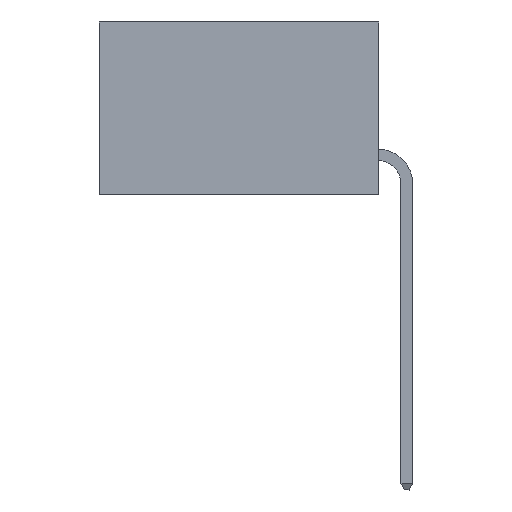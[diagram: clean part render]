
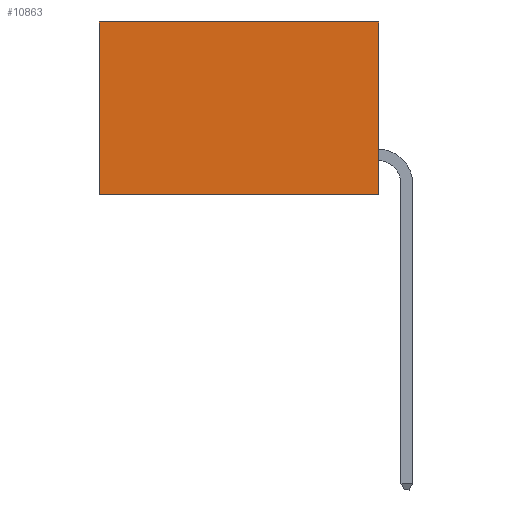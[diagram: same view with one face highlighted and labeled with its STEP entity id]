
A CAD part, left-side view. The second image highlights one B-rep face of the part: STEP entity #10863.
In plain terms, the highlighted planar face has unit normal (-1, 0, 0).
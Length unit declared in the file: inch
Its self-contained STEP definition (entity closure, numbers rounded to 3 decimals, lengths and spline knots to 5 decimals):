
#72 = CARTESIAN_POINT ( 'NONE',  ( 0.298, 0., -0.37 ) ) ;
#429 = DIRECTION ( 'NONE',  ( 0., 0., -1. ) ) ;
#1013 = VERTEX_POINT ( 'NONE', #72 ) ;
#1356 = VERTEX_POINT ( 'NONE', #2576 ) ;
#2576 = CARTESIAN_POINT ( 'NONE',  ( 0.298, 0.6, -0.37 ) ) ;
#2597 = DIRECTION ( 'NONE',  ( 0., 1., 0. ) ) ;
#3176 = VERTEX_POINT ( 'NONE', #16357 ) ;
#3367 = EDGE_CURVE ( 'NONE', #12695, #3176, #22529, .T. ) ;
#4934 = PLANE ( 'NONE',  #14690 ) ;
#4949 = EDGE_LOOP ( 'NONE', ( #16089, #23183, #5332, #28671 ) ) ;
#5332 = ORIENTED_EDGE ( 'NONE', *, *, #9638, .F. ) ;
#6008 = CARTESIAN_POINT ( 'NONE',  ( 0.298, 0., -0.37 ) ) ;
#7789 = DIRECTION ( 'NONE',  ( 0., 0., -1. ) ) ;
#9040 = VECTOR ( 'NONE', #7789, 39.37008 ) ;
#9498 = DIRECTION ( 'NONE',  ( 1., 0., 0. ) ) ;
#9638 = EDGE_CURVE ( 'NONE', #12695, #1013, #15044, .T. ) ;
#10863 = ADVANCED_FACE ( 'NONE', ( #22324 ), #4934, .F. ) ;
#12443 = VECTOR ( 'NONE', #15086, 39.37008 ) ;
#12695 = VERTEX_POINT ( 'NONE', #15808 ) ;
#14014 = EDGE_CURVE ( 'NONE', #1013, #1356, #24351, .T. ) ;
#14690 = AXIS2_PLACEMENT_3D ( 'NONE', #22974, #9498, #25219 ) ;
#15044 = LINE ( 'NONE', #16769, #9040 ) ;
#15086 = DIRECTION ( 'NONE',  ( 0., 1., 0. ) ) ;
#15808 = CARTESIAN_POINT ( 'NONE',  ( 0.298, 0., 0. ) ) ;
#16089 = ORIENTED_EDGE ( 'NONE', *, *, #26502, .T. ) ;
#16247 = CARTESIAN_POINT ( 'NONE',  ( 0.298, 0.6, 0. ) ) ;
#16357 = CARTESIAN_POINT ( 'NONE',  ( 0.298, 0.6, 0. ) ) ;
#16769 = CARTESIAN_POINT ( 'NONE',  ( 0.298, 0., 0. ) ) ;
#17192 = VECTOR ( 'NONE', #429, 39.37008 ) ;
#20768 = CARTESIAN_POINT ( 'NONE',  ( 0.298, 0., 0. ) ) ;
#22324 = FACE_OUTER_BOUND ( 'NONE', #4949, .T. ) ;
#22529 = LINE ( 'NONE', #20768, #23244 ) ;
#22974 = CARTESIAN_POINT ( 'NONE',  ( 0.298, 0., 0. ) ) ;
#23133 = LINE ( 'NONE', #16247, #17192 ) ;
#23183 = ORIENTED_EDGE ( 'NONE', *, *, #14014, .F. ) ;
#23244 = VECTOR ( 'NONE', #2597, 39.37008 ) ;
#24351 = LINE ( 'NONE', #6008, #12443 ) ;
#25219 = DIRECTION ( 'NONE',  ( 0., 0., -1. ) ) ;
#26502 = EDGE_CURVE ( 'NONE', #3176, #1356, #23133, .T. ) ;
#28671 = ORIENTED_EDGE ( 'NONE', *, *, #3367, .T. ) ;
